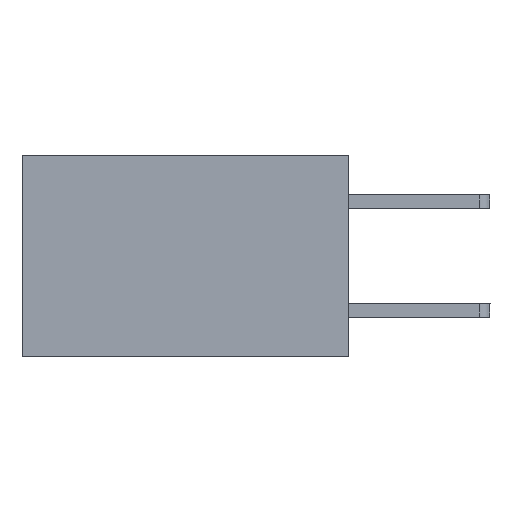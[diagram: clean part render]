
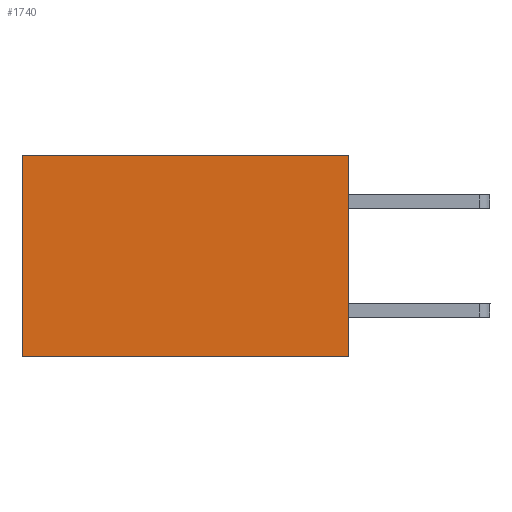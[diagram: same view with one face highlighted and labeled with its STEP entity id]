
A CAD part, left-side view. The second image highlights one B-rep face of the part: STEP entity #1740.
In plain terms, the highlighted planar face has unit normal (-1, 0, 0).
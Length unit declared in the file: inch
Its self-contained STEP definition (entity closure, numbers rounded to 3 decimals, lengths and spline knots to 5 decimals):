
#147 = VECTOR ( 'NONE', #5789, 39.37008 ) ;
#243 = VERTEX_POINT ( 'NONE', #10498 ) ;
#616 = EDGE_LOOP ( 'NONE', ( #5466, #10409, #9980, #6533 ) ) ;
#1387 = CARTESIAN_POINT ( 'NONE',  ( 0.298, 0.6, 0. ) ) ;
#1740 = ADVANCED_FACE ( 'NONE', ( #8211 ), #7353, .F. ) ;
#1974 = VERTEX_POINT ( 'NONE', #8920 ) ;
#2206 = LINE ( 'NONE', #5807, #5828 ) ;
#2311 = CARTESIAN_POINT ( 'NONE',  ( 0.298, 0., 0. ) ) ;
#2342 = DIRECTION ( 'NONE',  ( 0., 0., -1. ) ) ;
#2846 = CARTESIAN_POINT ( 'NONE',  ( 0.298, 0.6, -0.37 ) ) ;
#4856 = EDGE_CURVE ( 'NONE', #243, #5424, #6392, .T. ) ;
#5379 = VECTOR ( 'NONE', #7922, 39.37008 ) ;
#5424 = VERTEX_POINT ( 'NONE', #2846 ) ;
#5466 = ORIENTED_EDGE ( 'NONE', *, *, #5991, .T. ) ;
#5596 = CARTESIAN_POINT ( 'NONE',  ( 0.298, 0., -0.37 ) ) ;
#5733 = VECTOR ( 'NONE', #9993, 39.37008 ) ;
#5740 = VERTEX_POINT ( 'NONE', #1387 ) ;
#5789 = DIRECTION ( 'NONE',  ( 0., 1., 0. ) ) ;
#5807 = CARTESIAN_POINT ( 'NONE',  ( 0.298, 0.6, 0. ) ) ;
#5828 = VECTOR ( 'NONE', #10152, 39.37008 ) ;
#5991 = EDGE_CURVE ( 'NONE', #5740, #5424, #2206, .T. ) ;
#6392 = LINE ( 'NONE', #5596, #5733 ) ;
#6491 = DIRECTION ( 'NONE',  ( 1., 0., 0. ) ) ;
#6533 = ORIENTED_EDGE ( 'NONE', *, *, #10033, .T. ) ;
#6709 = AXIS2_PLACEMENT_3D ( 'NONE', #2311, #6491, #2342 ) ;
#7169 = CARTESIAN_POINT ( 'NONE',  ( 0.298, 0., 0. ) ) ;
#7353 = PLANE ( 'NONE',  #6709 ) ;
#7922 = DIRECTION ( 'NONE',  ( 0., 0., -1. ) ) ;
#8211 = FACE_OUTER_BOUND ( 'NONE', #616, .T. ) ;
#8216 = EDGE_CURVE ( 'NONE', #1974, #243, #8860, .T. ) ;
#8860 = LINE ( 'NONE', #7169, #5379 ) ;
#8920 = CARTESIAN_POINT ( 'NONE',  ( 0.298, 0., 0. ) ) ;
#9140 = LINE ( 'NONE', #10710, #147 ) ;
#9980 = ORIENTED_EDGE ( 'NONE', *, *, #8216, .F. ) ;
#9993 = DIRECTION ( 'NONE',  ( 0., 1., 0. ) ) ;
#10033 = EDGE_CURVE ( 'NONE', #1974, #5740, #9140, .T. ) ;
#10152 = DIRECTION ( 'NONE',  ( 0., 0., -1. ) ) ;
#10409 = ORIENTED_EDGE ( 'NONE', *, *, #4856, .F. ) ;
#10498 = CARTESIAN_POINT ( 'NONE',  ( 0.298, 0., -0.37 ) ) ;
#10710 = CARTESIAN_POINT ( 'NONE',  ( 0.298, 0., 0. ) ) ;
